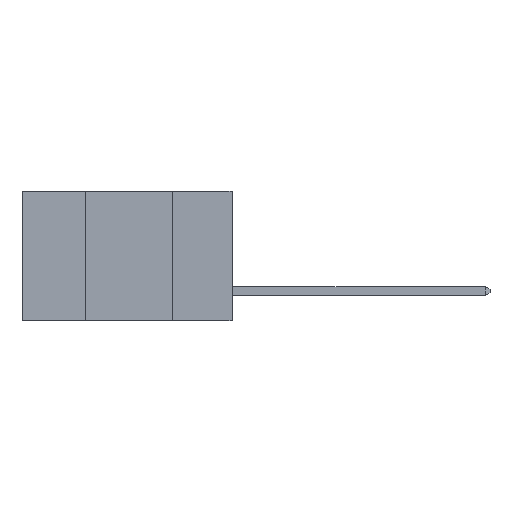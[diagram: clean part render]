
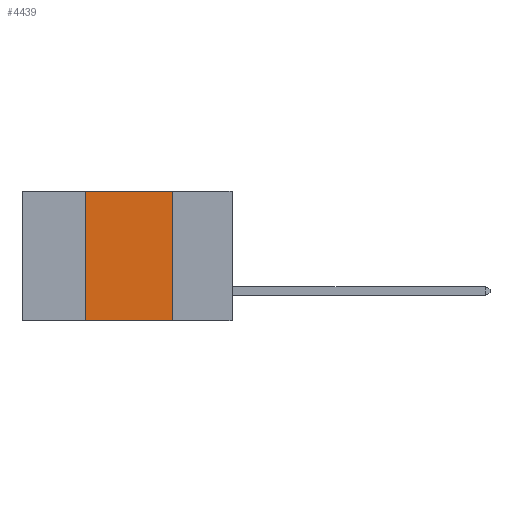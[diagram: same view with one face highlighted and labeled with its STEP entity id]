
A CAD part, left-side view. The second image highlights one B-rep face of the part: STEP entity #4439.
In plain terms, the highlighted planar face has unit normal (-1, 0, 0).
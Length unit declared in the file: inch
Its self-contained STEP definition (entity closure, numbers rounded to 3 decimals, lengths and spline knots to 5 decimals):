
#96 = PLANE ( 'NONE',  #5604 ) ;
#165 = ORIENTED_EDGE ( 'NONE', *, *, #1669, .T. ) ;
#265 = ORIENTED_EDGE ( 'NONE', *, *, #3991, .F. ) ;
#418 = CARTESIAN_POINT ( 'NONE',  ( 0., 0.6, -0.37 ) ) ;
#480 = VERTEX_POINT ( 'NONE', #2352 ) ;
#816 = CARTESIAN_POINT ( 'NONE',  ( 0., 0.42, 0. ) ) ;
#894 = DIRECTION ( 'NONE',  ( 0., 0., 1. ) ) ;
#1044 = CARTESIAN_POINT ( 'NONE',  ( 0., 0.6, 0. ) ) ;
#1322 = VERTEX_POINT ( 'NONE', #11233 ) ;
#1669 = EDGE_CURVE ( 'NONE', #1322, #480, #14596, .T. ) ;
#2057 = FACE_OUTER_BOUND ( 'NONE', #13093, .T. ) ;
#2140 = EDGE_CURVE ( 'NONE', #10940, #8051, #11244, .T. ) ;
#2351 = VECTOR ( 'NONE', #15118, 39.37008 ) ;
#2352 = CARTESIAN_POINT ( 'NONE',  ( 0., 0.17, -0.37 ) ) ;
#2821 = EDGE_CURVE ( 'NONE', #8051, #480, #9557, .T. ) ;
#3269 = LINE ( 'NONE', #816, #15412 ) ;
#3324 = DIRECTION ( 'NONE',  ( 0., 0., -1. ) ) ;
#3421 = DIRECTION ( 'NONE',  ( 1., 0., 0. ) ) ;
#3991 = EDGE_CURVE ( 'NONE', #1322, #10940, #3269, .T. ) ;
#4439 = ADVANCED_FACE ( 'NONE', ( #2057 ), #96, .F. ) ;
#4826 = VECTOR ( 'NONE', #13000, 39.37008 ) ;
#5604 = AXIS2_PLACEMENT_3D ( 'NONE', #1044, #3421, #3324 ) ;
#5833 = CARTESIAN_POINT ( 'NONE',  ( 0., 0.17, 0. ) ) ;
#6295 = VECTOR ( 'NONE', #11422, 39.37008 ) ;
#7189 = ORIENTED_EDGE ( 'NONE', *, *, #2140, .F. ) ;
#8051 = VERTEX_POINT ( 'NONE', #5833 ) ;
#9557 = LINE ( 'NONE', #12559, #6295 ) ;
#10937 = CARTESIAN_POINT ( 'NONE',  ( 0., 0.42, 0. ) ) ;
#10940 = VERTEX_POINT ( 'NONE', #10937 ) ;
#11233 = CARTESIAN_POINT ( 'NONE',  ( 0., 0.42, -0.37 ) ) ;
#11244 = LINE ( 'NONE', #13663, #4826 ) ;
#11422 = DIRECTION ( 'NONE',  ( 0., 0., -1. ) ) ;
#12559 = CARTESIAN_POINT ( 'NONE',  ( 0., 0.17, 0. ) ) ;
#13000 = DIRECTION ( 'NONE',  ( 0., -1., 0. ) ) ;
#13093 = EDGE_LOOP ( 'NONE', ( #14739, #7189, #265, #165 ) ) ;
#13663 = CARTESIAN_POINT ( 'NONE',  ( 0., 0.6, 0. ) ) ;
#14596 = LINE ( 'NONE', #418, #2351 ) ;
#14739 = ORIENTED_EDGE ( 'NONE', *, *, #2821, .F. ) ;
#15118 = DIRECTION ( 'NONE',  ( 0., -1., 0. ) ) ;
#15412 = VECTOR ( 'NONE', #894, 39.37008 ) ;
